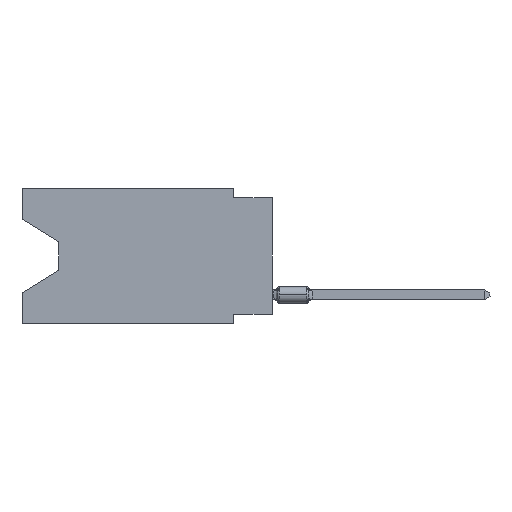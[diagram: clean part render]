
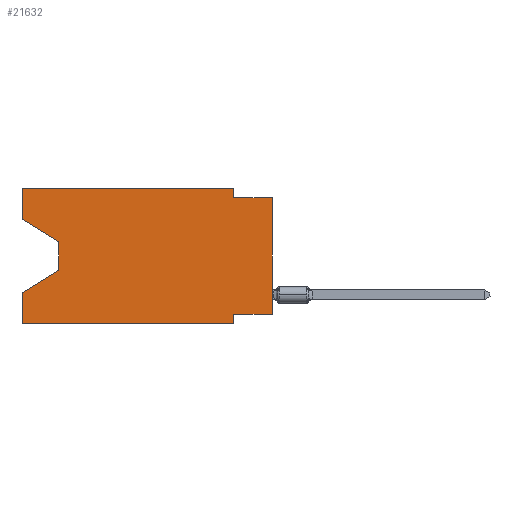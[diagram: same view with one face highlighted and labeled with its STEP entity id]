
A CAD part, left-side view. The second image highlights one B-rep face of the part: STEP entity #21632.
In plain terms, the highlighted planar face has unit normal (-1, 0, 0).
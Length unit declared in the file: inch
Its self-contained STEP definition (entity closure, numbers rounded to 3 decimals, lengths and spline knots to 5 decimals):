
#542 = DIRECTION ( 'NONE',  ( 0., 1., 0. ) ) ;
#1902 = VECTOR ( 'NONE', #8782, 39.37008 ) ;
#3115 = EDGE_CURVE ( 'NONE', #4952, #15466, #7705, .T. ) ;
#3197 = VECTOR ( 'NONE', #19581, 39.37008 ) ;
#3199 = CARTESIAN_POINT ( 'NONE',  ( 0., 0.645, -0.08025 ) ) ;
#3219 = VERTEX_POINT ( 'NONE', #10229 ) ;
#3303 = ORIENTED_EDGE ( 'NONE', *, *, #3115, .T. ) ;
#3904 = DIRECTION ( 'NONE',  ( 0., -1., 0. ) ) ;
#3917 = VECTOR ( 'NONE', #17677, 39.37008 ) ;
#4033 = LINE ( 'NONE', #14514, #3197 ) ;
#4408 = VECTOR ( 'NONE', #11103, 39.37008 ) ;
#4460 = EDGE_CURVE ( 'NONE', #12172, #4952, #18698, .T. ) ;
#4952 = VERTEX_POINT ( 'NONE', #6235 ) ;
#5248 = CARTESIAN_POINT ( 'NONE',  ( 0., 0., -0.025 ) ) ;
#5460 = LINE ( 'NONE', #9262, #3917 ) ;
#5674 = EDGE_CURVE ( 'NONE', #18129, #22464, #18810, .T. ) ;
#5867 = DIRECTION ( 'NONE',  ( 0., 0.855, -0.519 ) ) ;
#5975 = VECTOR ( 'NONE', #9932, 39.37008 ) ;
#6082 = ORIENTED_EDGE ( 'NONE', *, *, #20126, .F. ) ;
#6235 = CARTESIAN_POINT ( 'NONE',  ( 0., 0.55, -0.212 ) ) ;
#6626 = ORIENTED_EDGE ( 'NONE', *, *, #21033, .F. ) ;
#6729 = ORIENTED_EDGE ( 'NONE', *, *, #14733, .F. ) ;
#6880 = ORIENTED_EDGE ( 'NONE', *, *, #4460, .T. ) ;
#7073 = LINE ( 'NONE', #21142, #13858 ) ;
#7259 = ORIENTED_EDGE ( 'NONE', *, *, #18950, .T. ) ;
#7308 = AXIS2_PLACEMENT_3D ( 'NONE', #7880, #13183, #11443 ) ;
#7666 = ORIENTED_EDGE ( 'NONE', *, *, #14220, .F. ) ;
#7705 = LINE ( 'NONE', #14968, #12980 ) ;
#7880 = CARTESIAN_POINT ( 'NONE',  ( 0., 0.645, 0. ) ) ;
#7993 = DIRECTION ( 'NONE',  ( 0., 0., 1. ) ) ;
#8056 = ORIENTED_EDGE ( 'NONE', *, *, #19829, .F. ) ;
#8558 = ORIENTED_EDGE ( 'NONE', *, *, #20170, .T. ) ;
#8609 = CARTESIAN_POINT ( 'NONE',  ( 0., 0.1, -0.025 ) ) ;
#8782 = DIRECTION ( 'NONE',  ( 0., 0., -1. ) ) ;
#8902 = VECTOR ( 'NONE', #3904, 39.37008 ) ;
#9059 = DIRECTION ( 'NONE',  ( 0., 0., 1. ) ) ;
#9119 = DIRECTION ( 'NONE',  ( 0., 0., 1. ) ) ;
#9262 = CARTESIAN_POINT ( 'NONE',  ( 0., 0.645, -0.08025 ) ) ;
#9290 = CARTESIAN_POINT ( 'NONE',  ( 0., 0., -0.325 ) ) ;
#9500 = CARTESIAN_POINT ( 'NONE',  ( 0., 0.1, -0.35 ) ) ;
#9876 = VECTOR ( 'NONE', #9059, 39.37008 ) ;
#9932 = DIRECTION ( 'NONE',  ( 0., 0., -1. ) ) ;
#10051 = CARTESIAN_POINT ( 'NONE',  ( 0., 0., 0. ) ) ;
#10229 = CARTESIAN_POINT ( 'NONE',  ( 0., 0.1, -0.325 ) ) ;
#10432 = CARTESIAN_POINT ( 'NONE',  ( 0., 0., -0.325 ) ) ;
#10600 = ORIENTED_EDGE ( 'NONE', *, *, #5674, .T. ) ;
#10994 = LINE ( 'NONE', #21482, #4408 ) ;
#11103 = DIRECTION ( 'NONE',  ( 0., -1., 0. ) ) ;
#11121 = LINE ( 'NONE', #9290, #20477 ) ;
#11142 = VECTOR ( 'NONE', #9119, 39.37008 ) ;
#11157 = LINE ( 'NONE', #19693, #8902 ) ;
#11443 = DIRECTION ( 'NONE',  ( 0., 0., -1. ) ) ;
#12121 = VERTEX_POINT ( 'NONE', #3199 ) ;
#12172 = VERTEX_POINT ( 'NONE', #15854 ) ;
#12561 = LINE ( 'NONE', #17883, #11142 ) ;
#12980 = VECTOR ( 'NONE', #5867, 39.37008 ) ;
#13086 = VECTOR ( 'NONE', #7993, 39.37008 ) ;
#13183 = DIRECTION ( 'NONE',  ( 1., 0., 0. ) ) ;
#13749 = VERTEX_POINT ( 'NONE', #22194 ) ;
#13858 = VECTOR ( 'NONE', #22639, 39.37008 ) ;
#14220 = EDGE_CURVE ( 'NONE', #3219, #21460, #21009, .T. ) ;
#14506 = CARTESIAN_POINT ( 'NONE',  ( 0., 0.645, -0.35 ) ) ;
#14514 = CARTESIAN_POINT ( 'NONE',  ( 0., 0.645, -0.35 ) ) ;
#14733 = EDGE_CURVE ( 'NONE', #15875, #13749, #11157, .T. ) ;
#14753 = VERTEX_POINT ( 'NONE', #14506 ) ;
#14968 = CARTESIAN_POINT ( 'NONE',  ( 0., 0.55, -0.212 ) ) ;
#15466 = VERTEX_POINT ( 'NONE', #19271 ) ;
#15726 = EDGE_CURVE ( 'NONE', #14753, #15466, #12561, .T. ) ;
#15854 = CARTESIAN_POINT ( 'NONE',  ( 0., 0.55, -0.138 ) ) ;
#15875 = VERTEX_POINT ( 'NONE', #20870 ) ;
#15955 = EDGE_LOOP ( 'NONE', ( #8558, #6880, #3303, #18866, #7259, #7666, #8056, #10600, #16212, #6082, #6729, #6626 ) ) ;
#16212 = ORIENTED_EDGE ( 'NONE', *, *, #22638, .F. ) ;
#16361 = VERTEX_POINT ( 'NONE', #8609 ) ;
#16439 = LINE ( 'NONE', #21629, #9876 ) ;
#16622 = CARTESIAN_POINT ( 'NONE',  ( 0., 0.55, -0.138 ) ) ;
#16631 = PLANE ( 'NONE',  #7308 ) ;
#17677 = DIRECTION ( 'NONE',  ( 0., -0.855, -0.519 ) ) ;
#17883 = CARTESIAN_POINT ( 'NONE',  ( 0., 0.645, 0. ) ) ;
#18129 = VERTEX_POINT ( 'NONE', #10432 ) ;
#18698 = LINE ( 'NONE', #16622, #5975 ) ;
#18810 = LINE ( 'NONE', #10051, #13086 ) ;
#18866 = ORIENTED_EDGE ( 'NONE', *, *, #15726, .F. ) ;
#18950 = EDGE_CURVE ( 'NONE', #14753, #21460, #4033, .T. ) ;
#19271 = CARTESIAN_POINT ( 'NONE',  ( 0., 0.645, -0.26975 ) ) ;
#19581 = DIRECTION ( 'NONE',  ( 0., -1., 0. ) ) ;
#19693 = CARTESIAN_POINT ( 'NONE',  ( 0., 0.645, 0. ) ) ;
#19829 = EDGE_CURVE ( 'NONE', #18129, #3219, #11121, .T. ) ;
#20109 = FACE_OUTER_BOUND ( 'NONE', #15955, .T. ) ;
#20126 = EDGE_CURVE ( 'NONE', #13749, #16361, #7073, .T. ) ;
#20170 = EDGE_CURVE ( 'NONE', #12121, #12172, #5460, .T. ) ;
#20477 = VECTOR ( 'NONE', #542, 39.37008 ) ;
#20870 = CARTESIAN_POINT ( 'NONE',  ( 0., 0.645, 0. ) ) ;
#21009 = LINE ( 'NONE', #22613, #1902 ) ;
#21033 = EDGE_CURVE ( 'NONE', #12121, #15875, #16439, .T. ) ;
#21142 = CARTESIAN_POINT ( 'NONE',  ( 0., 0.1, 0. ) ) ;
#21460 = VERTEX_POINT ( 'NONE', #9500 ) ;
#21482 = CARTESIAN_POINT ( 'NONE',  ( 0., 0., -0.025 ) ) ;
#21629 = CARTESIAN_POINT ( 'NONE',  ( 0., 0.645, 0. ) ) ;
#21632 = ADVANCED_FACE ( 'NONE', ( #20109 ), #16631, .F. ) ;
#22194 = CARTESIAN_POINT ( 'NONE',  ( 0., 0.1, 0. ) ) ;
#22464 = VERTEX_POINT ( 'NONE', #5248 ) ;
#22613 = CARTESIAN_POINT ( 'NONE',  ( 0., 0.1, -0.35 ) ) ;
#22638 = EDGE_CURVE ( 'NONE', #16361, #22464, #10994, .T. ) ;
#22639 = DIRECTION ( 'NONE',  ( 0., 0., -1. ) ) ;
